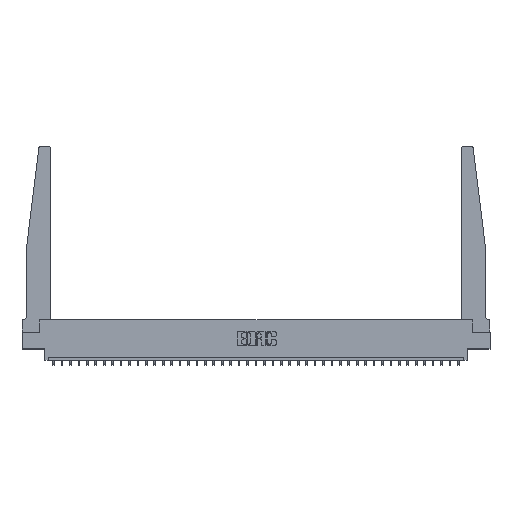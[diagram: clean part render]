
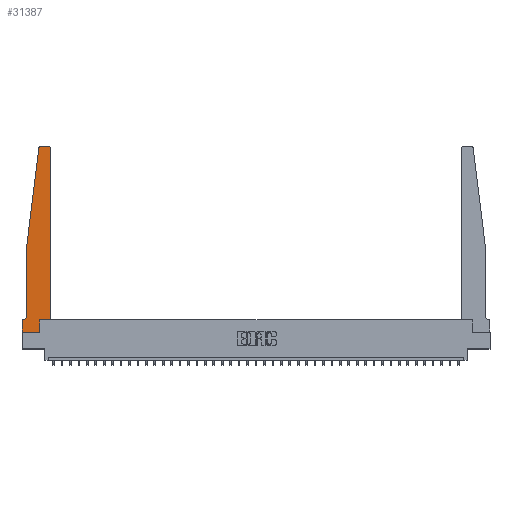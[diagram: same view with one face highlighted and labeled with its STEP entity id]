
A CAD part, top view. The second image highlights one B-rep face of the part: STEP entity #31387.
In plain terms, the highlighted planar face has unit normal (0, 0, 1).
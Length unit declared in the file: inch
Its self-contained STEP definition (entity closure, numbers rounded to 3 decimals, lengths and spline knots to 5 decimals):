
#411 = CARTESIAN_POINT ( 'NONE',  ( 0.065, 0.1875, 0.37 ) ) ;
#841 = EDGE_CURVE ( 'NONE', #17442, #24012, #1812, .T. ) ;
#934 = CARTESIAN_POINT ( 'NONE',  ( 0., 0., 0.37 ) ) ;
#1008 = AXIS2_PLACEMENT_3D ( 'NONE', #13736, #32197, #16403 ) ;
#1240 = LINE ( 'NONE', #934, #21617 ) ;
#1351 = CARTESIAN_POINT ( 'NONE',  ( 0.2605, 0., 0.37 ) ) ;
#1464 = DIRECTION ( 'NONE',  ( 1., 0., 0. ) ) ;
#1525 = FACE_OUTER_BOUND ( 'NONE', #11914, .T. ) ;
#1635 = ORIENTED_EDGE ( 'NONE', *, *, #16709, .T. ) ;
#1812 = LINE ( 'NONE', #19882, #29256 ) ;
#2118 = CARTESIAN_POINT ( 'NONE',  ( 0., 0., 0.37 ) ) ;
#2582 = CARTESIAN_POINT ( 'NONE',  ( 0.425, 2.72, 0.37 ) ) ;
#2656 = AXIS2_PLACEMENT_3D ( 'NONE', #33291, #17449, #1464 ) ;
#2752 = CARTESIAN_POINT ( 'NONE',  ( 0.425, 0.18, 0.37 ) ) ;
#3221 = DIRECTION ( 'NONE',  ( 0., 0., 1. ) ) ;
#3309 = ORIENTED_EDGE ( 'NONE', *, *, #31972, .T. ) ;
#4057 = VECTOR ( 'NONE', #19468, 39.37008 ) ;
#4422 = CARTESIAN_POINT ( 'NONE',  ( 0.065, 1.25, 0.37 ) ) ;
#4965 = ORIENTED_EDGE ( 'NONE', *, *, #16040, .T. ) ;
#5062 = LINE ( 'NONE', #2118, #32511 ) ;
#5760 = DIRECTION ( 'NONE',  ( -1., 0., 0. ) ) ;
#5895 = DIRECTION ( 'NONE',  ( 1., 0., 0. ) ) ;
#6083 = LINE ( 'NONE', #11041, #12387 ) ;
#6093 = LINE ( 'NONE', #11885, #32679 ) ;
#8717 = VERTEX_POINT ( 'NONE', #11542 ) ;
#8787 = CARTESIAN_POINT ( 'NONE',  ( 0.425, 0.18, 0.37 ) ) ;
#10229 = DIRECTION ( 'NONE',  ( 0., -1., 0. ) ) ;
#10322 = ORIENTED_EDGE ( 'NONE', *, *, #22611, .T. ) ;
#10402 = AXIS2_PLACEMENT_3D ( 'NONE', #19202, #21825, #5895 ) ;
#10478 = EDGE_CURVE ( 'NONE', #12393, #17550, #22470, .T. ) ;
#10749 = DIRECTION ( 'NONE',  ( 1., 0., 0. ) ) ;
#10946 = EDGE_CURVE ( 'NONE', #13844, #20518, #1240, .T. ) ;
#11041 = CARTESIAN_POINT ( 'NONE',  ( 0.2605, 0.18, 0.37 ) ) ;
#11331 = CARTESIAN_POINT ( 'NONE',  ( 0.065, 0.2375, 0.37 ) ) ;
#11335 = VERTEX_POINT ( 'NONE', #11331 ) ;
#11377 = CARTESIAN_POINT ( 'NONE',  ( 0.2605, 0.18, 0.37 ) ) ;
#11444 = CIRCLE ( 'NONE', #33965, 0.03 ) ;
#11542 = CARTESIAN_POINT ( 'NONE',  ( 0., 0.1875, 0.37 ) ) ;
#11840 = CARTESIAN_POINT ( 'NONE',  ( 0.065, 1.25, 0.37 ) ) ;
#11885 = CARTESIAN_POINT ( 'NONE',  ( 0.065, 1.25, 0.37 ) ) ;
#11914 = EDGE_LOOP ( 'NONE', ( #30594, #10322, #32257, #11995, #15038, #1635, #16706, #30726, #3309, #4965, #18704, #34439 ) ) ;
#11995 = ORIENTED_EDGE ( 'NONE', *, *, #20459, .T. ) ;
#12387 = VECTOR ( 'NONE', #26862, 39.37008 ) ;
#12393 = VERTEX_POINT ( 'NONE', #21310 ) ;
#13736 = CARTESIAN_POINT ( 'NONE',  ( 0.015, 0.2375, 0.37 ) ) ;
#13844 = VERTEX_POINT ( 'NONE', #16902 ) ;
#14111 = VERTEX_POINT ( 'NONE', #15827 ) ;
#15038 = ORIENTED_EDGE ( 'NONE', *, *, #20873, .T. ) ;
#15308 = CIRCLE ( 'NONE', #1008, 0.05 ) ;
#15583 = EDGE_CURVE ( 'NONE', #31869, #17442, #18135, .T. ) ;
#15827 = CARTESIAN_POINT ( 'NONE',  ( 0.425, 0.18, 0.37 ) ) ;
#16040 = EDGE_CURVE ( 'NONE', #28649, #14111, #29674, .T. ) ;
#16403 = DIRECTION ( 'NONE',  ( -1., 0., 0. ) ) ;
#16476 = VECTOR ( 'NONE', #10749, 39.37008 ) ;
#16706 = ORIENTED_EDGE ( 'NONE', *, *, #17162, .T. ) ;
#16709 = EDGE_CURVE ( 'NONE', #18797, #8717, #31700, .T. ) ;
#16842 = CARTESIAN_POINT ( 'NONE',  ( 0.395, 2.75, 0.37 ) ) ;
#16902 = CARTESIAN_POINT ( 'NONE',  ( 0., 0., 0.37 ) ) ;
#17162 = EDGE_CURVE ( 'NONE', #8717, #13844, #5062, .T. ) ;
#17442 = VERTEX_POINT ( 'NONE', #16842 ) ;
#17449 = DIRECTION ( 'NONE',  ( 0., 0., 1. ) ) ;
#17550 = VERTEX_POINT ( 'NONE', #11840 ) ;
#17642 = VECTOR ( 'NONE', #5760, 39.37008 ) ;
#18135 = CIRCLE ( 'NONE', #2656, 0.03 ) ;
#18594 = CARTESIAN_POINT ( 'NONE',  ( 0.015, 0.1875, 0.37 ) ) ;
#18704 = ORIENTED_EDGE ( 'NONE', *, *, #30841, .T. ) ;
#18797 = VERTEX_POINT ( 'NONE', #18594 ) ;
#19202 = CARTESIAN_POINT ( 'NONE',  ( 0., 0.1875, 0.37 ) ) ;
#19216 = CARTESIAN_POINT ( 'NONE',  ( 0.27653, 2.72, 0.37 ) ) ;
#19468 = DIRECTION ( 'NONE',  ( 0., 1., 0. ) ) ;
#19882 = CARTESIAN_POINT ( 'NONE',  ( 0.25, 2.75, 0.37 ) ) ;
#20387 = DIRECTION ( 'NONE',  ( -0.122, -0.992, 0. ) ) ;
#20459 = EDGE_CURVE ( 'NONE', #17550, #11335, #6093, .T. ) ;
#20518 = VERTEX_POINT ( 'NONE', #1351 ) ;
#20873 = EDGE_CURVE ( 'NONE', #11335, #18797, #15308, .T. ) ;
#21310 = CARTESIAN_POINT ( 'NONE',  ( 0.24675, 2.72367, 0.37 ) ) ;
#21617 = VECTOR ( 'NONE', #24874, 39.37008 ) ;
#21825 = DIRECTION ( 'NONE',  ( 0., 0., 1. ) ) ;
#21837 = DIRECTION ( 'NONE',  ( 1., 0., 0. ) ) ;
#22470 = LINE ( 'NONE', #4422, #28692 ) ;
#22611 = EDGE_CURVE ( 'NONE', #24012, #12393, #11444, .T. ) ;
#24012 = VERTEX_POINT ( 'NONE', #26348 ) ;
#24874 = DIRECTION ( 'NONE',  ( 1., 0., 0. ) ) ;
#25280 = LINE ( 'NONE', #8787, #4057 ) ;
#26348 = CARTESIAN_POINT ( 'NONE',  ( 0.27653, 2.75, 0.37 ) ) ;
#26862 = DIRECTION ( 'NONE',  ( 0., 1., 0. ) ) ;
#27702 = DIRECTION ( 'NONE',  ( 0., -1., 0. ) ) ;
#27718 = DIRECTION ( 'NONE',  ( -1., 0., 0. ) ) ;
#28649 = VERTEX_POINT ( 'NONE', #11377 ) ;
#28692 = VECTOR ( 'NONE', #20387, 39.37008 ) ;
#29256 = VECTOR ( 'NONE', #27718, 39.37008 ) ;
#29674 = LINE ( 'NONE', #2752, #16476 ) ;
#29706 = PLANE ( 'NONE',  #10402 ) ;
#30594 = ORIENTED_EDGE ( 'NONE', *, *, #841, .T. ) ;
#30726 = ORIENTED_EDGE ( 'NONE', *, *, #10946, .T. ) ;
#30841 = EDGE_CURVE ( 'NONE', #14111, #31869, #25280, .T. ) ;
#31387 = ADVANCED_FACE ( 'NONE', ( #1525 ), #29706, .T. ) ;
#31700 = LINE ( 'NONE', #411, #17642 ) ;
#31869 = VERTEX_POINT ( 'NONE', #2582 ) ;
#31972 = EDGE_CURVE ( 'NONE', #20518, #28649, #6083, .T. ) ;
#32197 = DIRECTION ( 'NONE',  ( 0., 0., -1. ) ) ;
#32257 = ORIENTED_EDGE ( 'NONE', *, *, #10478, .T. ) ;
#32511 = VECTOR ( 'NONE', #10229, 39.37008 ) ;
#32679 = VECTOR ( 'NONE', #27702, 39.37008 ) ;
#33291 = CARTESIAN_POINT ( 'NONE',  ( 0.395, 2.72, 0.37 ) ) ;
#33965 = AXIS2_PLACEMENT_3D ( 'NONE', #19216, #3221, #21837 ) ;
#34439 = ORIENTED_EDGE ( 'NONE', *, *, #15583, .T. ) ;
